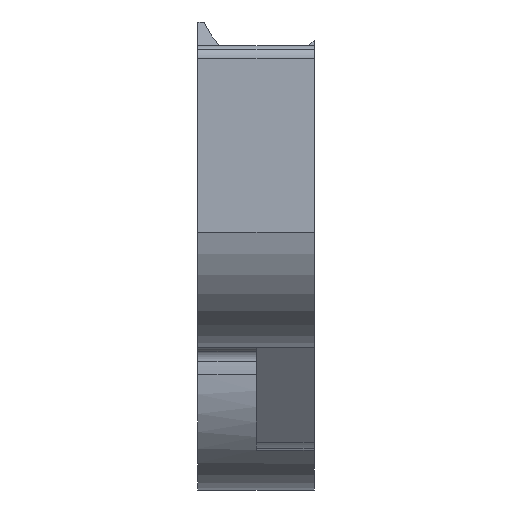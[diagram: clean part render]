
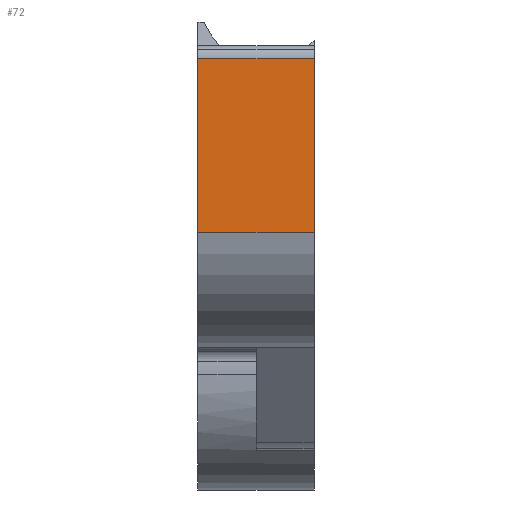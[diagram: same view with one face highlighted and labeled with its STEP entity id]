
A CAD part, left-side view. The second image highlights one B-rep face of the part: STEP entity #72.
In plain terms, the highlighted planar face has unit normal (-1, 0, 0).
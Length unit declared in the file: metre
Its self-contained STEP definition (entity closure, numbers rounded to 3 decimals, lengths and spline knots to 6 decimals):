
#72=ADVANCED_FACE('0:54526',(#141),#142,.F.);
#141=FACE_OUTER_BOUND('',#234,.T.);
#142=PLANE('',#235);
#234=EDGE_LOOP('',(#467,#468,#469,#470));
#235=AXIS2_PLACEMENT_3D('',#471,#472,#473);
#467=ORIENTED_EDGE('',*,*,#704,.F.);
#468=ORIENTED_EDGE('',*,*,#757,.T.);
#469=ORIENTED_EDGE('',*,*,#765,.F.);
#470=ORIENTED_EDGE('',*,*,#766,.F.);
#471=CARTESIAN_POINT('',(-0.138325,0.0236,-0.012385));
#472=DIRECTION('',(1.0,0.,0.0));
#473=DIRECTION('',(0.,-1.0,0.0));
#704=EDGE_CURVE('0:54736',#858,#860,#861,.T.);
#757=EDGE_CURVE('0:54709',#858,#951,#953,.F.);
#765=EDGE_CURVE('0:54739',#963,#951,#964,.T.);
#766=EDGE_CURVE('0:54742',#860,#963,#965,.F.);
#858=VERTEX_POINT('',#1086);
#860=VERTEX_POINT('',#1088);
#861=LINE('',#1089,#1090);
#951=VERTEX_POINT('',#1206);
#953=LINE('',#1208,#1209);
#963=VERTEX_POINT('',#1223);
#964=LINE('',#1224,#1225);
#965=LINE('',#1226,#1227);
#1086=CARTESIAN_POINT('',(-0.138325,0.02865,-0.00613));
#1088=CARTESIAN_POINT('',(-0.138325,0.0196,-0.00613));
#1089=CARTESIAN_POINT('',(-0.138325,0.0256,-0.00613));
#1090=VECTOR('',#1366,0.00905);
#1206=CARTESIAN_POINT('',(-0.138325,0.02865,-0.01964));
#1208=CARTESIAN_POINT('',(-0.138325,0.02865,-0.016707));
#1209=VECTOR('',#1471,0.01351);
#1223=CARTESIAN_POINT('',(-0.138325,0.0196,-0.01964));
#1224=CARTESIAN_POINT('',(-0.138325,0.02865,-0.01964));
#1225=VECTOR('',#1485,0.00905);
#1226=CARTESIAN_POINT('',(-0.138325,0.0196,-0.014154));
#1227=VECTOR('',#1486,0.01351);
#1366=DIRECTION('',(0.,-1.0,0.0));
#1471=DIRECTION('',(0.0,0.0,1.0));
#1485=DIRECTION('',(0.,1.0,0.0));
#1486=DIRECTION('',(0.0,0.0,1.0));
